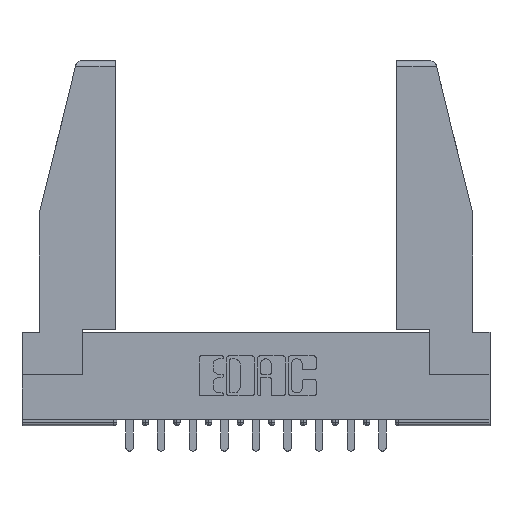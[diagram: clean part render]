
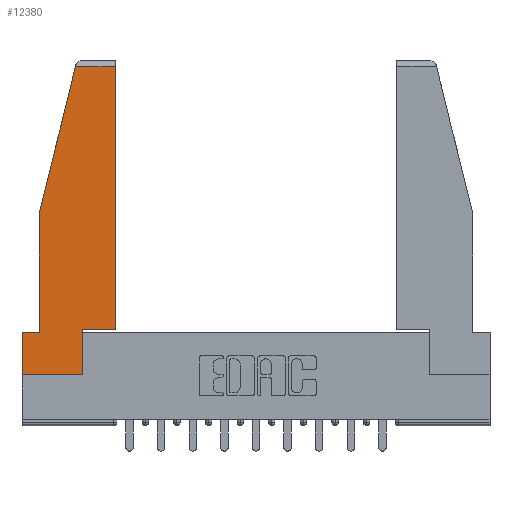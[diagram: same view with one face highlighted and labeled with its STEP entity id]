
A CAD part, top view. The second image highlights one B-rep face of the part: STEP entity #12380.
In plain terms, the highlighted planar face has unit normal (0, 0, 1).
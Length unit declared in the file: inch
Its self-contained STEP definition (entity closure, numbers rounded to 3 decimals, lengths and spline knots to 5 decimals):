
#11 = LINE ( 'NONE', #5910, #3083 ) ;
#169 = DIRECTION ( 'NONE',  ( 0., 0., 1. ) ) ;
#190 = VECTOR ( 'NONE', #13960, 39.37008 ) ;
#261 = LINE ( 'NONE', #6234, #5870 ) ;
#649 = CARTESIAN_POINT ( 'NONE',  ( 0.297, 0., 0. ) ) ;
#711 = EDGE_CURVE ( 'NONE', #14392, #5067, #5561, .T. ) ;
#787 = ORIENTED_EDGE ( 'NONE', *, *, #711, .T. ) ;
#1241 = VERTEX_POINT ( 'NONE', #11337 ) ;
#1385 = DIRECTION ( 'NONE',  ( 1., 0., 0. ) ) ;
#1492 = AXIS2_PLACEMENT_3D ( 'NONE', #10491, #169, #11705 ) ;
#1969 = ORIENTED_EDGE ( 'NONE', *, *, #14106, .T. ) ;
#2112 = CARTESIAN_POINT ( 'NONE',  ( 0., 0.21, 0. ) ) ;
#2526 = VERTEX_POINT ( 'NONE', #6937 ) ;
#2779 = EDGE_CURVE ( 'NONE', #4452, #1241, #261, .T. ) ;
#2789 = CARTESIAN_POINT ( 'NONE',  ( 0.461, 1.52, 0. ) ) ;
#2848 = EDGE_CURVE ( 'NONE', #1241, #8150, #4242, .T. ) ;
#3029 = LINE ( 'NONE', #12350, #5020 ) ;
#3052 = CARTESIAN_POINT ( 'NONE',  ( 0., 0.21, 0. ) ) ;
#3083 = VECTOR ( 'NONE', #1385, 39.37008 ) ;
#3199 = CARTESIAN_POINT ( 'NONE',  ( 0.086, 0.21, 0. ) ) ;
#3315 = DIRECTION ( 'NONE',  ( 0., 1., 0. ) ) ;
#3627 = VECTOR ( 'NONE', #13684, 39.37008 ) ;
#3823 = VECTOR ( 'NONE', #14680, 39.37008 ) ;
#4019 = DIRECTION ( 'NONE',  ( 1., 0., 0. ) ) ;
#4020 = LINE ( 'NONE', #9909, #11515 ) ;
#4242 = LINE ( 'NONE', #649, #3627 ) ;
#4279 = DIRECTION ( 'NONE',  ( -1., 0., 0. ) ) ;
#4452 = VERTEX_POINT ( 'NONE', #9143 ) ;
#4543 = LINE ( 'NONE', #8342, #12497 ) ;
#4840 = EDGE_CURVE ( 'NONE', #9116, #14392, #8965, .T. ) ;
#5020 = VECTOR ( 'NONE', #6546, 39.37008 ) ;
#5067 = VERTEX_POINT ( 'NONE', #3052 ) ;
#5356 = EDGE_CURVE ( 'NONE', #9952, #5899, #9625, .T. ) ;
#5395 = ORIENTED_EDGE ( 'NONE', *, *, #4840, .T. ) ;
#5561 = LINE ( 'NONE', #2112, #12448 ) ;
#5755 = FACE_OUTER_BOUND ( 'NONE', #10817, .T. ) ;
#5843 = EDGE_CURVE ( 'NONE', #5899, #9116, #4020, .T. ) ;
#5870 = VECTOR ( 'NONE', #4019, 39.37008 ) ;
#5899 = VERTEX_POINT ( 'NONE', #14241 ) ;
#5910 = CARTESIAN_POINT ( 'NONE',  ( 0.297, 0.223, 0. ) ) ;
#6234 = CARTESIAN_POINT ( 'NONE',  ( 0., 0., 0. ) ) ;
#6412 = ORIENTED_EDGE ( 'NONE', *, *, #2779, .T. ) ;
#6546 = DIRECTION ( 'NONE',  ( 0., -1., 0. ) ) ;
#6937 = CARTESIAN_POINT ( 'NONE',  ( 0.461, 0.223, 0. ) ) ;
#7073 = ORIENTED_EDGE ( 'NONE', *, *, #5843, .T. ) ;
#8140 = PLANE ( 'NONE',  #1492 ) ;
#8150 = VERTEX_POINT ( 'NONE', #12045 ) ;
#8272 = EDGE_CURVE ( 'NONE', #5067, #4452, #3029, .T. ) ;
#8342 = CARTESIAN_POINT ( 'NONE',  ( 0.461, 0.223, 0. ) ) ;
#8965 = LINE ( 'NONE', #12408, #3823 ) ;
#9059 = EDGE_CURVE ( 'NONE', #8150, #2526, #11, .T. ) ;
#9116 = VERTEX_POINT ( 'NONE', #11929 ) ;
#9143 = CARTESIAN_POINT ( 'NONE',  ( 0., 0., 0. ) ) ;
#9311 = CARTESIAN_POINT ( 'NONE',  ( 0., 1.52, 0. ) ) ;
#9625 = LINE ( 'NONE', #9311, #190 ) ;
#9909 = CARTESIAN_POINT ( 'NONE',  ( 0.271, 1.55, 0. ) ) ;
#9952 = VERTEX_POINT ( 'NONE', #2789 ) ;
#10491 = CARTESIAN_POINT ( 'NONE',  ( 0., 0., 0. ) ) ;
#10817 = EDGE_LOOP ( 'NONE', ( #1969, #12112, #7073, #5395, #787, #11868, #6412, #13351, #13012 ) ) ;
#11337 = CARTESIAN_POINT ( 'NONE',  ( 0.297, 0., 0. ) ) ;
#11515 = VECTOR ( 'NONE', #14381, 39.37008 ) ;
#11705 = DIRECTION ( 'NONE',  ( 1., 0., 0. ) ) ;
#11868 = ORIENTED_EDGE ( 'NONE', *, *, #8272, .T. ) ;
#11929 = CARTESIAN_POINT ( 'NONE',  ( 0.086, 0.8, 0. ) ) ;
#12045 = CARTESIAN_POINT ( 'NONE',  ( 0.297, 0.223, 0. ) ) ;
#12112 = ORIENTED_EDGE ( 'NONE', *, *, #5356, .T. ) ;
#12350 = CARTESIAN_POINT ( 'NONE',  ( 0., 0.21, 0. ) ) ;
#12380 = ADVANCED_FACE ( 'NONE', ( #5755 ), #8140, .T. ) ;
#12408 = CARTESIAN_POINT ( 'NONE',  ( 0.086, 0.8, 0. ) ) ;
#12448 = VECTOR ( 'NONE', #4279, 39.37008 ) ;
#12497 = VECTOR ( 'NONE', #3315, 39.37008 ) ;
#13012 = ORIENTED_EDGE ( 'NONE', *, *, #9059, .T. ) ;
#13351 = ORIENTED_EDGE ( 'NONE', *, *, #2848, .T. ) ;
#13684 = DIRECTION ( 'NONE',  ( 0., 1., 0. ) ) ;
#13960 = DIRECTION ( 'NONE',  ( -1., 0., 0. ) ) ;
#14106 = EDGE_CURVE ( 'NONE', #2526, #9952, #4543, .T. ) ;
#14241 = CARTESIAN_POINT ( 'NONE',  ( 0.2636, 1.52, 0. ) ) ;
#14381 = DIRECTION ( 'NONE',  ( -0.239, -0.971, 0. ) ) ;
#14392 = VERTEX_POINT ( 'NONE', #3199 ) ;
#14680 = DIRECTION ( 'NONE',  ( 0., -1., 0. ) ) ;
